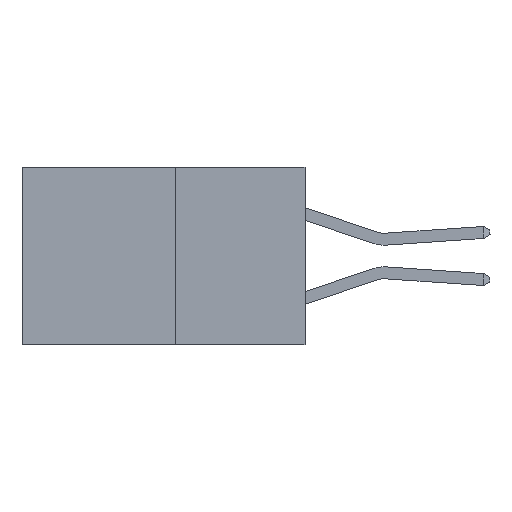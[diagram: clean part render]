
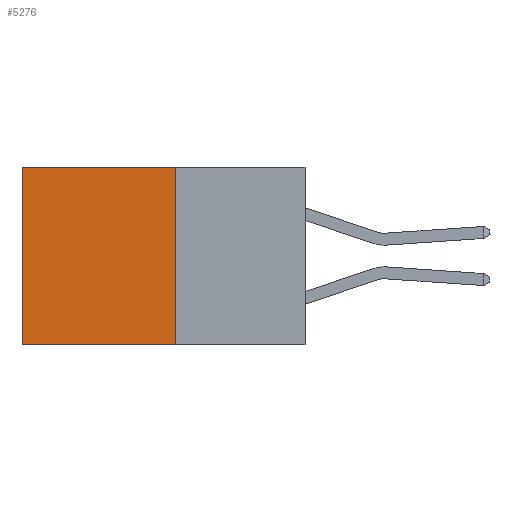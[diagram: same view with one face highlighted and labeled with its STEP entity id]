
A CAD part, left-side view. The second image highlights one B-rep face of the part: STEP entity #5276.
In plain terms, the highlighted planar face has unit normal (-1, 0, 0).
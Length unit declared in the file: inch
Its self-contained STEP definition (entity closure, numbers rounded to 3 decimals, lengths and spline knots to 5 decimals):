
#5 = VECTOR ( 'NONE', #10181, 39.37008 ) ;
#324 = LINE ( 'NONE', #1412, #5 ) ;
#1017 = DIRECTION ( 'NONE',  ( 0., 1., 0. ) ) ;
#1090 = PLANE ( 'NONE',  #9864 ) ;
#1412 = CARTESIAN_POINT ( 'NONE',  ( 0.277, 0.27, -0.37 ) ) ;
#1476 = ORIENTED_EDGE ( 'NONE', *, *, #2399, .F. ) ;
#1872 = EDGE_CURVE ( 'NONE', #4158, #7857, #324, .T. ) ;
#2226 = EDGE_CURVE ( 'NONE', #9602, #6699, #8239, .T. ) ;
#2399 = EDGE_CURVE ( 'NONE', #9602, #4158, #10213, .T. ) ;
#3736 = ORIENTED_EDGE ( 'NONE', *, *, #4969, .T. ) ;
#3822 = DIRECTION ( 'NONE',  ( 1., 0., 0. ) ) ;
#4052 = EDGE_LOOP ( 'NONE', ( #3736, #9757, #1476, #4108 ) ) ;
#4108 = ORIENTED_EDGE ( 'NONE', *, *, #2226, .T. ) ;
#4148 = DIRECTION ( 'NONE',  ( 0., 0., -1. ) ) ;
#4158 = VERTEX_POINT ( 'NONE', #9808 ) ;
#4306 = CARTESIAN_POINT ( 'NONE',  ( 0.277, 0.59, -0.37 ) ) ;
#4349 = VECTOR ( 'NONE', #4148, 39.37008 ) ;
#4736 = CARTESIAN_POINT ( 'NONE',  ( 0.277, 0.59, -0.37 ) ) ;
#4969 = EDGE_CURVE ( 'NONE', #6699, #7857, #6971, .T. ) ;
#5276 = ADVANCED_FACE ( 'NONE', ( #7333 ), #1090, .F. ) ;
#6699 = VERTEX_POINT ( 'NONE', #6941 ) ;
#6941 = CARTESIAN_POINT ( 'NONE',  ( 0.277, 0.59, 0. ) ) ;
#6971 = LINE ( 'NONE', #4306, #9067 ) ;
#7333 = FACE_OUTER_BOUND ( 'NONE', #4052, .T. ) ;
#7857 = VERTEX_POINT ( 'NONE', #4736 ) ;
#7945 = CARTESIAN_POINT ( 'NONE',  ( 0.277, 0.27, 0. ) ) ;
#7986 = VECTOR ( 'NONE', #1017, 39.37008 ) ;
#8162 = DIRECTION ( 'NONE',  ( 0., 0., -1. ) ) ;
#8239 = LINE ( 'NONE', #8383, #7986 ) ;
#8383 = CARTESIAN_POINT ( 'NONE',  ( 0.277, 0.27, 0. ) ) ;
#8481 = CARTESIAN_POINT ( 'NONE',  ( 0.277, 0.27, -0.37 ) ) ;
#8799 = CARTESIAN_POINT ( 'NONE',  ( 0.277, 0.27, -0.37 ) ) ;
#9067 = VECTOR ( 'NONE', #8162, 39.37008 ) ;
#9266 = DIRECTION ( 'NONE',  ( 0., 0., -1. ) ) ;
#9602 = VERTEX_POINT ( 'NONE', #7945 ) ;
#9757 = ORIENTED_EDGE ( 'NONE', *, *, #1872, .F. ) ;
#9808 = CARTESIAN_POINT ( 'NONE',  ( 0.277, 0.27, -0.37 ) ) ;
#9864 = AXIS2_PLACEMENT_3D ( 'NONE', #8481, #3822, #9266 ) ;
#10181 = DIRECTION ( 'NONE',  ( 0., 1., 0. ) ) ;
#10213 = LINE ( 'NONE', #8799, #4349 ) ;
